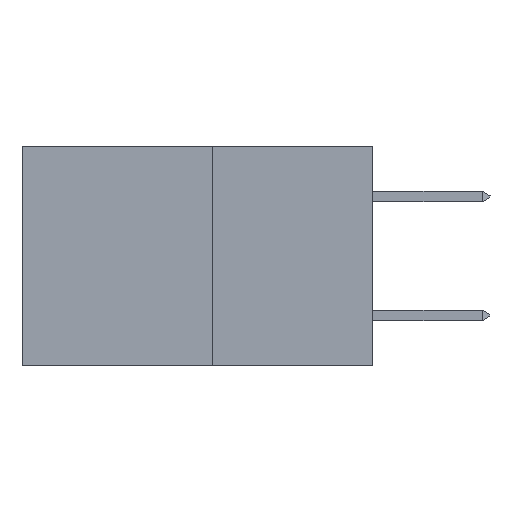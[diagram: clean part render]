
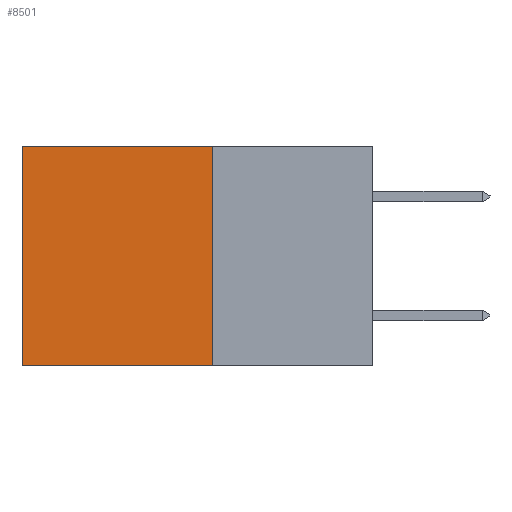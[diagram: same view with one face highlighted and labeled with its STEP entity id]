
A CAD part, left-side view. The second image highlights one B-rep face of the part: STEP entity #8501.
In plain terms, the highlighted planar face has unit normal (-1, 0, 0).
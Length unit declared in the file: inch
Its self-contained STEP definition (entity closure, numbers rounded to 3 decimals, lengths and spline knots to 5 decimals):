
#629 = EDGE_CURVE ( 'NONE', #5690, #913, #2340, .T. ) ;
#913 = VERTEX_POINT ( 'NONE', #4341 ) ;
#1315 = PLANE ( 'NONE',  #11043 ) ;
#2340 = LINE ( 'NONE', #21220, #23861 ) ;
#2676 = ORIENTED_EDGE ( 'NONE', *, *, #629, .F. ) ;
#3353 = CARTESIAN_POINT ( 'NONE',  ( 0.277, 0.59, -0.37 ) ) ;
#4341 = CARTESIAN_POINT ( 'NONE',  ( 0.277, 0.27, -0.37 ) ) ;
#5460 = DIRECTION ( 'NONE',  ( 0., 0., -1. ) ) ;
#5690 = VERTEX_POINT ( 'NONE', #16751 ) ;
#5762 = EDGE_LOOP ( 'NONE', ( #25153, #17173, #2676, #14281 ) ) ;
#5777 = DIRECTION ( 'NONE',  ( 0., 1., 0. ) ) ;
#6815 = EDGE_CURVE ( 'NONE', #913, #18208, #19440, .T. ) ;
#6994 = FACE_OUTER_BOUND ( 'NONE', #5762, .T. ) ;
#8017 = DIRECTION ( 'NONE',  ( 0., 1., 0. ) ) ;
#8101 = EDGE_CURVE ( 'NONE', #5690, #19251, #20632, .T. ) ;
#8500 = VECTOR ( 'NONE', #23594, 39.37008 ) ;
#8501 = ADVANCED_FACE ( 'NONE', ( #6994 ), #1315, .F. ) ;
#9861 = VECTOR ( 'NONE', #8017, 39.37008 ) ;
#10072 = LINE ( 'NONE', #3353, #8500 ) ;
#10393 = CARTESIAN_POINT ( 'NONE',  ( 0.277, 0.59, -0.37 ) ) ;
#11043 = AXIS2_PLACEMENT_3D ( 'NONE', #15504, #17556, #5460 ) ;
#14281 = ORIENTED_EDGE ( 'NONE', *, *, #8101, .T. ) ;
#15504 = CARTESIAN_POINT ( 'NONE',  ( 0.277, 0.27, -0.37 ) ) ;
#16454 = DIRECTION ( 'NONE',  ( 0., 0., -1. ) ) ;
#16751 = CARTESIAN_POINT ( 'NONE',  ( 0.277, 0.27, 0. ) ) ;
#17094 = EDGE_CURVE ( 'NONE', #19251, #18208, #10072, .T. ) ;
#17173 = ORIENTED_EDGE ( 'NONE', *, *, #6815, .F. ) ;
#17556 = DIRECTION ( 'NONE',  ( 1., 0., 0. ) ) ;
#17882 = CARTESIAN_POINT ( 'NONE',  ( 0.277, 0.27, -0.37 ) ) ;
#18208 = VERTEX_POINT ( 'NONE', #10393 ) ;
#19251 = VERTEX_POINT ( 'NONE', #19481 ) ;
#19440 = LINE ( 'NONE', #17882, #24121 ) ;
#19481 = CARTESIAN_POINT ( 'NONE',  ( 0.277, 0.59, 0. ) ) ;
#20632 = LINE ( 'NONE', #22165, #9861 ) ;
#21220 = CARTESIAN_POINT ( 'NONE',  ( 0.277, 0.27, -0.37 ) ) ;
#22165 = CARTESIAN_POINT ( 'NONE',  ( 0.277, 0.27, 0. ) ) ;
#23594 = DIRECTION ( 'NONE',  ( 0., 0., -1. ) ) ;
#23861 = VECTOR ( 'NONE', #16454, 39.37008 ) ;
#24121 = VECTOR ( 'NONE', #5777, 39.37008 ) ;
#25153 = ORIENTED_EDGE ( 'NONE', *, *, #17094, .T. ) ;
